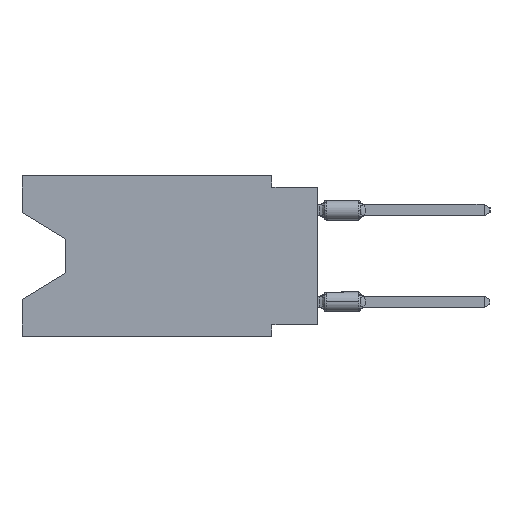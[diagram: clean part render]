
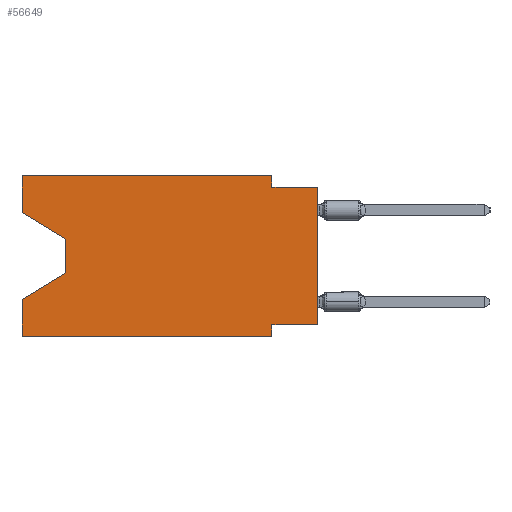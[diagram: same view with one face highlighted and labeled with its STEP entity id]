
A CAD part, left-side view. The second image highlights one B-rep face of the part: STEP entity #56649.
In plain terms, the highlighted planar face has unit normal (-1, 0, 0).
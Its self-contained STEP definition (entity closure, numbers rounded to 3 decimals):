
#621 = ORIENTED_EDGE ( 'NONE', *, *, #36913, .F. ) ;
#875 = LINE ( 'NONE', #20196, #55900 ) ;
#926 = DIRECTION ( 'NONE',  ( 0., -1., 0. ) ) ;
#943 = VERTEX_POINT ( 'NONE', #4991 ) ;
#2087 = EDGE_CURVE ( 'NONE', #54241, #43400, #2149, .T. ) ;
#2149 = LINE ( 'NONE', #21476, #17443 ) ;
#2422 = DIRECTION ( 'NONE',  ( 1., 0., 0. ) ) ;
#3205 = VERTEX_POINT ( 'NONE', #42207 ) ;
#4366 = VERTEX_POINT ( 'NONE', #22077 ) ;
#4983 = DIRECTION ( 'NONE',  ( 0., 0., -1. ) ) ;
#4991 = CARTESIAN_POINT ( 'NONE',  ( 0., 16.383, -6.852 ) ) ;
#5446 = CARTESIAN_POINT ( 'NONE',  ( 0., 0., -0.635 ) ) ;
#5489 = AXIS2_PLACEMENT_3D ( 'NONE', #30985, #2422, #6546 ) ;
#6546 = DIRECTION ( 'NONE',  ( 0., 0., -1. ) ) ;
#6824 = DIRECTION ( 'NONE',  ( 0., 0., 1. ) ) ;
#7158 = FACE_OUTER_BOUND ( 'NONE', #54981, .T. ) ;
#8006 = VERTEX_POINT ( 'NONE', #40256 ) ;
#8237 = ORIENTED_EDGE ( 'NONE', *, *, #9986, .T. ) ;
#8802 = DIRECTION ( 'NONE',  ( 0., 0., -1. ) ) ;
#9227 = VECTOR ( 'NONE', #30016, 1000. ) ;
#9986 = EDGE_CURVE ( 'NONE', #54241, #52368, #23378, .T. ) ;
#10044 = CARTESIAN_POINT ( 'NONE',  ( 0., 0., -0.635 ) ) ;
#11158 = EDGE_CURVE ( 'NONE', #29153, #52368, #28915, .T. ) ;
#12869 = CARTESIAN_POINT ( 'NONE',  ( 0., 2.54, -8.255 ) ) ;
#13062 = EDGE_CURVE ( 'NONE', #4366, #29153, #13235, .T. ) ;
#13235 = LINE ( 'NONE', #13551, #19213 ) ;
#13551 = CARTESIAN_POINT ( 'NONE',  ( 0., 2.54, 0. ) ) ;
#15695 = EDGE_CURVE ( 'NONE', #43400, #27658, #875, .T. ) ;
#17443 = VECTOR ( 'NONE', #20540, 1000. ) ;
#18277 = CARTESIAN_POINT ( 'NONE',  ( 0., 2.54, -8.89 ) ) ;
#18863 = VERTEX_POINT ( 'NONE', #21451 ) ;
#18889 = EDGE_CURVE ( 'NONE', #18863, #8006, #50286, .T. ) ;
#19213 = VECTOR ( 'NONE', #8802, 1000. ) ;
#20196 = CARTESIAN_POINT ( 'NONE',  ( 0., 2.54, -8.89 ) ) ;
#20540 = DIRECTION ( 'NONE',  ( 0., 1., 0. ) ) ;
#21451 = CARTESIAN_POINT ( 'NONE',  ( 0., 13.97, -3.505 ) ) ;
#21476 = CARTESIAN_POINT ( 'NONE',  ( 0., 0., -8.255 ) ) ;
#22077 = CARTESIAN_POINT ( 'NONE',  ( 0., 2.54, 0. ) ) ;
#22343 = CARTESIAN_POINT ( 'NONE',  ( 0., 13.97, -5.385 ) ) ;
#23378 = LINE ( 'NONE', #57896, #34310 ) ;
#24367 = CARTESIAN_POINT ( 'NONE',  ( 0., 2.54, -0.635 ) ) ;
#25014 = LINE ( 'NONE', #44341, #62225 ) ;
#25097 = EDGE_CURVE ( 'NONE', #3205, #27658, #25014, .T. ) ;
#25890 = LINE ( 'NONE', #45222, #9227 ) ;
#26204 = CARTESIAN_POINT ( 'NONE',  ( 0., 13.97, -3.505 ) ) ;
#26611 = EDGE_CURVE ( 'NONE', #8006, #943, #56240, .T. ) ;
#26628 = EDGE_CURVE ( 'NONE', #31914, #4366, #48291, .T. ) ;
#27098 = CARTESIAN_POINT ( 'NONE',  ( 0., 16.383, 0. ) ) ;
#27658 = VERTEX_POINT ( 'NONE', #18277 ) ;
#28915 = LINE ( 'NONE', #5446, #56684 ) ;
#29153 = VERTEX_POINT ( 'NONE', #24367 ) ;
#29932 = VECTOR ( 'NONE', #53038, 1000. ) ;
#30016 = DIRECTION ( 'NONE',  ( 0., 0., 1. ) ) ;
#30985 = CARTESIAN_POINT ( 'NONE',  ( 0., 16.383, 0. ) ) ;
#31354 = ORIENTED_EDGE ( 'NONE', *, *, #48573, .F. ) ;
#31490 = CARTESIAN_POINT ( 'NONE',  ( 0., 0., -8.255 ) ) ;
#31698 = ORIENTED_EDGE ( 'NONE', *, *, #61387, .T. ) ;
#31914 = VERTEX_POINT ( 'NONE', #27098 ) ;
#32778 = DIRECTION ( 'NONE',  ( 0., -0.855, -0.519 ) ) ;
#34003 = VECTOR ( 'NONE', #61897, 1000. ) ;
#34310 = VECTOR ( 'NONE', #57276, 1000. ) ;
#35597 = ORIENTED_EDGE ( 'NONE', *, *, #25097, .T. ) ;
#36602 = LINE ( 'NONE', #47034, #60881 ) ;
#36913 = EDGE_CURVE ( 'NONE', #3205, #943, #61503, .T. ) ;
#38828 = ORIENTED_EDGE ( 'NONE', *, *, #11158, .F. ) ;
#38941 = ORIENTED_EDGE ( 'NONE', *, *, #18889, .T. ) ;
#39373 = VERTEX_POINT ( 'NONE', #52926 ) ;
#40256 = CARTESIAN_POINT ( 'NONE',  ( 0., 13.97, -5.385 ) ) ;
#41050 = CARTESIAN_POINT ( 'NONE',  ( 0., 16.383, 0. ) ) ;
#41955 = ORIENTED_EDGE ( 'NONE', *, *, #15695, .F. ) ;
#42207 = CARTESIAN_POINT ( 'NONE',  ( 0., 16.383, -8.89 ) ) ;
#43400 = VERTEX_POINT ( 'NONE', #12869 ) ;
#44341 = CARTESIAN_POINT ( 'NONE',  ( 0., 16.383, -8.89 ) ) ;
#44449 = ORIENTED_EDGE ( 'NONE', *, *, #13062, .F. ) ;
#45222 = CARTESIAN_POINT ( 'NONE',  ( 0., 16.383, 0. ) ) ;
#45231 = DIRECTION ( 'NONE',  ( 0., 0., -1. ) ) ;
#45836 = PLANE ( 'NONE',  #5489 ) ;
#47034 = CARTESIAN_POINT ( 'NONE',  ( 0., 16.383, -2.038 ) ) ;
#48291 = LINE ( 'NONE', #62522, #29932 ) ;
#48573 = EDGE_CURVE ( 'NONE', #39373, #31914, #25890, .T. ) ;
#49731 = ORIENTED_EDGE ( 'NONE', *, *, #2087, .F. ) ;
#50286 = LINE ( 'NONE', #26204, #59190 ) ;
#52368 = VERTEX_POINT ( 'NONE', #10044 ) ;
#52926 = CARTESIAN_POINT ( 'NONE',  ( 0., 16.383, -2.038 ) ) ;
#53038 = DIRECTION ( 'NONE',  ( 0., -1., 0. ) ) ;
#53604 = DIRECTION ( 'NONE',  ( 0., -1., 0. ) ) ;
#54241 = VERTEX_POINT ( 'NONE', #31490 ) ;
#54476 = ORIENTED_EDGE ( 'NONE', *, *, #26628, .F. ) ;
#54981 = EDGE_LOOP ( 'NONE', ( #31698, #38941, #59411, #621, #35597, #41955, #49731, #8237, #38828, #44449, #54476, #31354 ) ) ;
#55900 = VECTOR ( 'NONE', #4983, 1000. ) ;
#56240 = LINE ( 'NONE', #22343, #34003 ) ;
#56649 = ADVANCED_FACE ( 'NONE', ( #7158 ), #45836, .F. ) ;
#56684 = VECTOR ( 'NONE', #53604, 1000. ) ;
#57276 = DIRECTION ( 'NONE',  ( 0., 0., 1. ) ) ;
#57896 = CARTESIAN_POINT ( 'NONE',  ( 0., 0., 0. ) ) ;
#59112 = VECTOR ( 'NONE', #6824, 1000. ) ;
#59190 = VECTOR ( 'NONE', #45231, 1000. ) ;
#59411 = ORIENTED_EDGE ( 'NONE', *, *, #26611, .T. ) ;
#60881 = VECTOR ( 'NONE', #32778, 1000. ) ;
#61387 = EDGE_CURVE ( 'NONE', #39373, #18863, #36602, .T. ) ;
#61503 = LINE ( 'NONE', #41050, #59112 ) ;
#61897 = DIRECTION ( 'NONE',  ( 0., 0.855, -0.519 ) ) ;
#62225 = VECTOR ( 'NONE', #926, 1000. ) ;
#62522 = CARTESIAN_POINT ( 'NONE',  ( 0., 16.383, 0. ) ) ;
